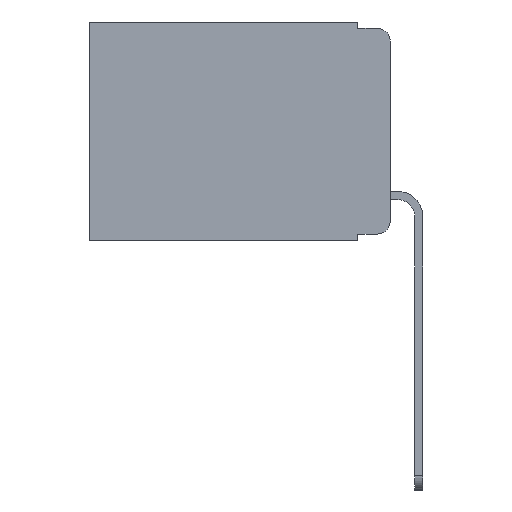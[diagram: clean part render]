
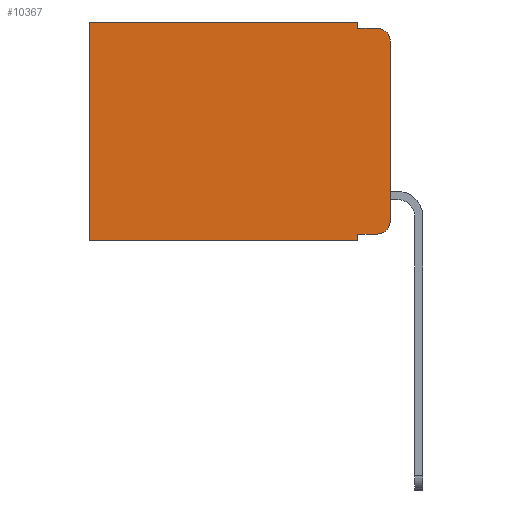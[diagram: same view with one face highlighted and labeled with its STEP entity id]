
A CAD part, left-side view. The second image highlights one B-rep face of the part: STEP entity #10367.
In plain terms, the highlighted planar face has unit normal (-1, 0, 0).
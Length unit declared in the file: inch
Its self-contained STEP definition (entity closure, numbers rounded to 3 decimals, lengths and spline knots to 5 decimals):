
#187 = ORIENTED_EDGE ( 'NONE', *, *, #2975, .F. ) ;
#401 = ORIENTED_EDGE ( 'NONE', *, *, #12527, .F. ) ;
#490 = CIRCLE ( 'NONE', #8052, 0.02 ) ;
#523 = DIRECTION ( 'NONE',  ( 0., 0., -1. ) ) ;
#553 = EDGE_CURVE ( 'NONE', #612, #6649, #7923, .T. ) ;
#612 = VERTEX_POINT ( 'NONE', #8009 ) ;
#1044 = EDGE_CURVE ( 'NONE', #6868, #2062, #3126, .T. ) ;
#1071 = VECTOR ( 'NONE', #7843, 39.37008 ) ;
#1165 = EDGE_CURVE ( 'NONE', #10010, #6663, #5317, .T. ) ;
#1198 = CARTESIAN_POINT ( 'NONE',  ( 0.298, 0.02, -0.333 ) ) ;
#1595 = FACE_OUTER_BOUND ( 'NONE', #8390, .T. ) ;
#1629 = DIRECTION ( 'NONE',  ( -1., 0., 0. ) ) ;
#1825 = LINE ( 'NONE', #5141, #12741 ) ;
#2062 = VERTEX_POINT ( 'NONE', #1198 ) ;
#2114 = CARTESIAN_POINT ( 'NONE',  ( 0.298, 0., 0. ) ) ;
#2159 = CARTESIAN_POINT ( 'NONE',  ( 0.298, 0., 0. ) ) ;
#2161 = DIRECTION ( 'NONE',  ( 0., 1., 0. ) ) ;
#2176 = EDGE_CURVE ( 'NONE', #2062, #6663, #490, .T. ) ;
#2394 = VECTOR ( 'NONE', #13556, 39.37008 ) ;
#2500 = CARTESIAN_POINT ( 'NONE',  ( 0.298, 0.02, -0.313 ) ) ;
#2598 = CIRCLE ( 'NONE', #7307, 0.02 ) ;
#2975 = EDGE_CURVE ( 'NONE', #5862, #6109, #5278, .T. ) ;
#3020 = CARTESIAN_POINT ( 'NONE',  ( 0.298, 0.02, -0.01 ) ) ;
#3126 = LINE ( 'NONE', #4182, #2394 ) ;
#3248 = DIRECTION ( 'NONE',  ( 0., 0., -1. ) ) ;
#3528 = CARTESIAN_POINT ( 'NONE',  ( 0.298, 0.051, -0.333 ) ) ;
#3843 = CARTESIAN_POINT ( 'NONE',  ( 0.298, 0., -0.313 ) ) ;
#3882 = CARTESIAN_POINT ( 'NONE',  ( 0.298, 0.02, -0.03 ) ) ;
#4182 = CARTESIAN_POINT ( 'NONE',  ( 0.298, 0.051, -0.333 ) ) ;
#4224 = ORIENTED_EDGE ( 'NONE', *, *, #9397, .T. ) ;
#4386 = DIRECTION ( 'NONE',  ( 0., 1., 0. ) ) ;
#5141 = CARTESIAN_POINT ( 'NONE',  ( 0.298, 0.051, 0. ) ) ;
#5278 = LINE ( 'NONE', #6692, #13258 ) ;
#5317 = LINE ( 'NONE', #14920, #1071 ) ;
#5437 = AXIS2_PLACEMENT_3D ( 'NONE', #2159, #10426, #11615 ) ;
#5862 = VERTEX_POINT ( 'NONE', #14347 ) ;
#5898 = VECTOR ( 'NONE', #4386, 39.37008 ) ;
#6109 = VERTEX_POINT ( 'NONE', #3020 ) ;
#6411 = EDGE_CURVE ( 'NONE', #11617, #14995, #6716, .T. ) ;
#6630 = ORIENTED_EDGE ( 'NONE', *, *, #1044, .T. ) ;
#6649 = VERTEX_POINT ( 'NONE', #10989 ) ;
#6663 = VERTEX_POINT ( 'NONE', #3843 ) ;
#6692 = CARTESIAN_POINT ( 'NONE',  ( 0.298, 0.051, -0.01 ) ) ;
#6716 = LINE ( 'NONE', #2114, #8604 ) ;
#6794 = ORIENTED_EDGE ( 'NONE', *, *, #15248, .F. ) ;
#6868 = VERTEX_POINT ( 'NONE', #3528 ) ;
#7307 = AXIS2_PLACEMENT_3D ( 'NONE', #3882, #1629, #7443 ) ;
#7443 = DIRECTION ( 'NONE',  ( 0., 0., -1. ) ) ;
#7586 = CARTESIAN_POINT ( 'NONE',  ( 0.298, 0.473, 0. ) ) ;
#7843 = DIRECTION ( 'NONE',  ( 0., 0., -1. ) ) ;
#7923 = LINE ( 'NONE', #8062, #5898 ) ;
#8009 = CARTESIAN_POINT ( 'NONE',  ( 0.298, 0.051, -0.343 ) ) ;
#8052 = AXIS2_PLACEMENT_3D ( 'NONE', #2500, #12009, #13302 ) ;
#8062 = CARTESIAN_POINT ( 'NONE',  ( 0.298, 0., -0.343 ) ) ;
#8390 = EDGE_LOOP ( 'NONE', ( #9584, #4224, #187, #6794, #9634, #14750, #9484, #401, #6630, #10994 ) ) ;
#8604 = VECTOR ( 'NONE', #2161, 39.37008 ) ;
#8721 = EDGE_CURVE ( 'NONE', #14995, #6649, #14262, .T. ) ;
#8792 = DIRECTION ( 'NONE',  ( 0., 0., -1. ) ) ;
#9233 = PLANE ( 'NONE',  #5437 ) ;
#9397 = EDGE_CURVE ( 'NONE', #10010, #6109, #2598, .T. ) ;
#9484 = ORIENTED_EDGE ( 'NONE', *, *, #553, .F. ) ;
#9584 = ORIENTED_EDGE ( 'NONE', *, *, #1165, .F. ) ;
#9634 = ORIENTED_EDGE ( 'NONE', *, *, #6411, .T. ) ;
#10010 = VERTEX_POINT ( 'NONE', #12053 ) ;
#10367 = ADVANCED_FACE ( 'NONE', ( #1595 ), #9233, .F. ) ;
#10426 = DIRECTION ( 'NONE',  ( 1., 0., 0. ) ) ;
#10989 = CARTESIAN_POINT ( 'NONE',  ( 0.298, 0.473, -0.343 ) ) ;
#10994 = ORIENTED_EDGE ( 'NONE', *, *, #2176, .T. ) ;
#11272 = CARTESIAN_POINT ( 'NONE',  ( 0.298, 0.473, 0. ) ) ;
#11615 = DIRECTION ( 'NONE',  ( 0., 0., -1. ) ) ;
#11617 = VERTEX_POINT ( 'NONE', #14455 ) ;
#11725 = CARTESIAN_POINT ( 'NONE',  ( 0.298, 0.051, 0. ) ) ;
#11886 = VECTOR ( 'NONE', #3248, 39.37008 ) ;
#12009 = DIRECTION ( 'NONE',  ( -1., 0., 0. ) ) ;
#12053 = CARTESIAN_POINT ( 'NONE',  ( 0.298, 0., -0.03 ) ) ;
#12527 = EDGE_CURVE ( 'NONE', #6868, #612, #14637, .T. ) ;
#12544 = DIRECTION ( 'NONE',  ( 0., -1., 0. ) ) ;
#12741 = VECTOR ( 'NONE', #8792, 39.37008 ) ;
#12985 = VECTOR ( 'NONE', #523, 39.37008 ) ;
#13258 = VECTOR ( 'NONE', #12544, 39.37008 ) ;
#13302 = DIRECTION ( 'NONE',  ( 0., 0., -1. ) ) ;
#13556 = DIRECTION ( 'NONE',  ( 0., -1., 0. ) ) ;
#14262 = LINE ( 'NONE', #7586, #12985 ) ;
#14347 = CARTESIAN_POINT ( 'NONE',  ( 0.298, 0.051, -0.01 ) ) ;
#14455 = CARTESIAN_POINT ( 'NONE',  ( 0.298, 0.051, 0. ) ) ;
#14637 = LINE ( 'NONE', #11725, #11886 ) ;
#14750 = ORIENTED_EDGE ( 'NONE', *, *, #8721, .T. ) ;
#14920 = CARTESIAN_POINT ( 'NONE',  ( 0.298, 0., 0. ) ) ;
#14995 = VERTEX_POINT ( 'NONE', #11272 ) ;
#15248 = EDGE_CURVE ( 'NONE', #11617, #5862, #1825, .T. ) ;
